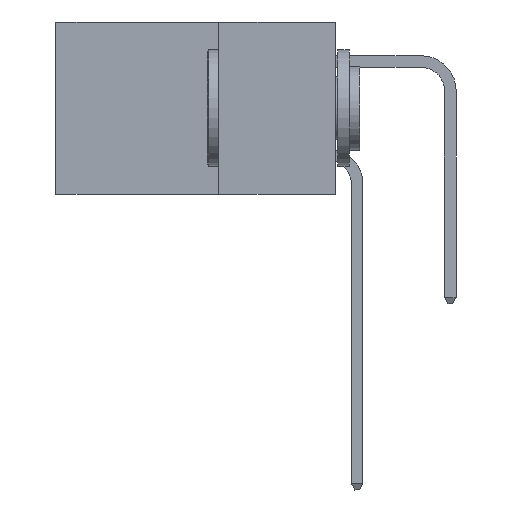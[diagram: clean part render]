
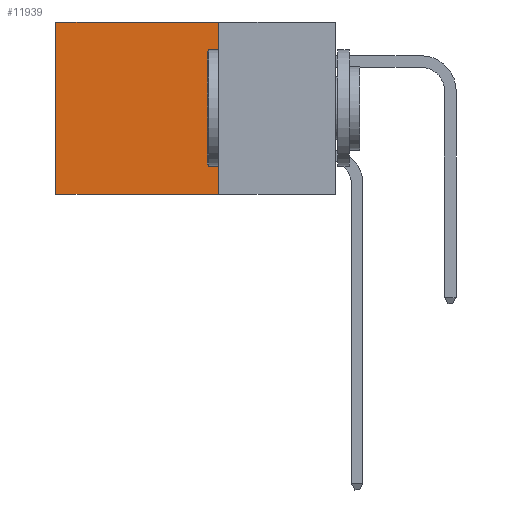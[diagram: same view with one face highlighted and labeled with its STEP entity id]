
A CAD part, left-side view. The second image highlights one B-rep face of the part: STEP entity #11939.
In plain terms, the highlighted planar face has unit normal (-1, 0, 0).
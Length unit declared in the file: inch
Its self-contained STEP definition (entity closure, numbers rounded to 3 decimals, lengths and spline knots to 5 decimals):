
#597 = CARTESIAN_POINT ( 'NONE',  ( 0.2875, 0.25, 0. ) ) ;
#3818 = AXIS2_PLACEMENT_3D ( 'NONE', #34809, #21321, #10837 ) ;
#4297 = EDGE_CURVE ( 'NONE', #6462, #21134, #19450, .T. ) ;
#4530 = DIRECTION ( 'NONE',  ( 0., 0., -1. ) ) ;
#5283 = VECTOR ( 'NONE', #26092, 39.37008 ) ;
#6462 = VERTEX_POINT ( 'NONE', #29541 ) ;
#10113 = LINE ( 'NONE', #11694, #5283 ) ;
#10837 = DIRECTION ( 'NONE',  ( 0., 0., -1. ) ) ;
#11606 = CARTESIAN_POINT ( 'NONE',  ( 0.2875, 0.6, -0.37 ) ) ;
#11694 = CARTESIAN_POINT ( 'NONE',  ( 0.2875, 0.25, 0. ) ) ;
#11939 = ADVANCED_FACE ( 'NONE', ( #16883 ), #31377, .F. ) ;
#14677 = VECTOR ( 'NONE', #28781, 39.37008 ) ;
#15964 = VECTOR ( 'NONE', #4530, 39.37008 ) ;
#16515 = CARTESIAN_POINT ( 'NONE',  ( 0.2875, 0.25, -0.37 ) ) ;
#16883 = FACE_OUTER_BOUND ( 'NONE', #42430, .T. ) ;
#18388 = CARTESIAN_POINT ( 'NONE',  ( 0.2875, 0.25, -0.37 ) ) ;
#18958 = CARTESIAN_POINT ( 'NONE',  ( 0.2875, 0.25, 0. ) ) ;
#19450 = LINE ( 'NONE', #38963, #14677 ) ;
#21134 = VERTEX_POINT ( 'NONE', #11606 ) ;
#21321 = DIRECTION ( 'NONE',  ( 1., 0., 0. ) ) ;
#21520 = DIRECTION ( 'NONE',  ( 0., 1., 0. ) ) ;
#25056 = LINE ( 'NONE', #597, #15964 ) ;
#26092 = DIRECTION ( 'NONE',  ( 0., 1., 0. ) ) ;
#28781 = DIRECTION ( 'NONE',  ( 0., 0., -1. ) ) ;
#29210 = ORIENTED_EDGE ( 'NONE', *, *, #38563, .F. ) ;
#29541 = CARTESIAN_POINT ( 'NONE',  ( 0.2875, 0.6, 0. ) ) ;
#31164 = LINE ( 'NONE', #18388, #33863 ) ;
#31377 = PLANE ( 'NONE',  #3818 ) ;
#31638 = ORIENTED_EDGE ( 'NONE', *, *, #4297, .T. ) ;
#32013 = ORIENTED_EDGE ( 'NONE', *, *, #37953, .T. ) ;
#33863 = VECTOR ( 'NONE', #21520, 39.37008 ) ;
#34809 = CARTESIAN_POINT ( 'NONE',  ( 0.2875, 0.25, 0. ) ) ;
#37246 = VERTEX_POINT ( 'NONE', #18958 ) ;
#37953 = EDGE_CURVE ( 'NONE', #37246, #6462, #10113, .T. ) ;
#38179 = VERTEX_POINT ( 'NONE', #16515 ) ;
#38563 = EDGE_CURVE ( 'NONE', #37246, #38179, #25056, .T. ) ;
#38963 = CARTESIAN_POINT ( 'NONE',  ( 0.2875, 0.6, 0. ) ) ;
#40746 = EDGE_CURVE ( 'NONE', #38179, #21134, #31164, .T. ) ;
#41367 = ORIENTED_EDGE ( 'NONE', *, *, #40746, .F. ) ;
#42430 = EDGE_LOOP ( 'NONE', ( #31638, #41367, #29210, #32013 ) ) ;
